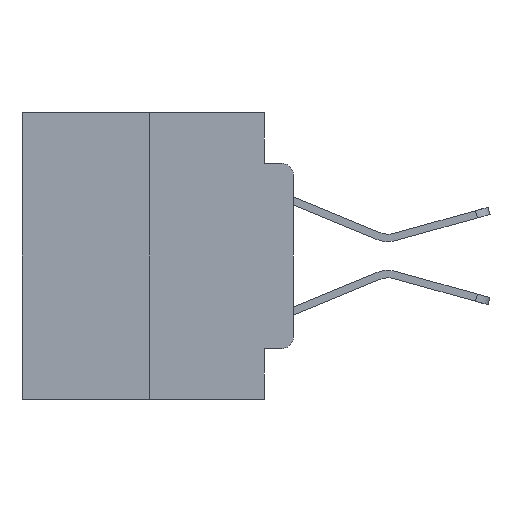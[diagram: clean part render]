
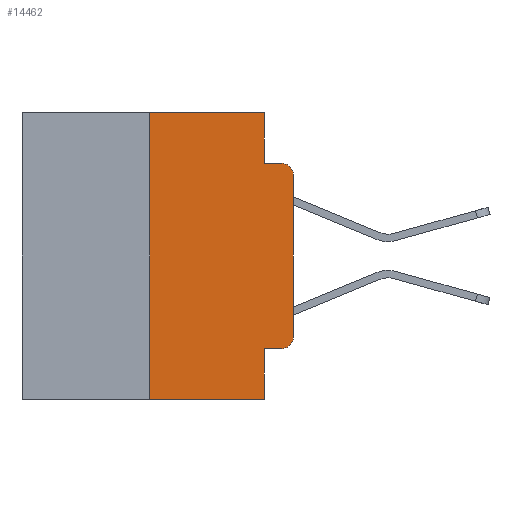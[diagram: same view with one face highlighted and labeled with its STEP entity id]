
A CAD part, left-side view. The second image highlights one B-rep face of the part: STEP entity #14462.
In plain terms, the highlighted planar face has unit normal (-1, 0, 0).
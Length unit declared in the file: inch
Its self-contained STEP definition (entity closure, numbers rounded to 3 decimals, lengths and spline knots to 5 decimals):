
#27 = EDGE_CURVE ( 'NONE', #13425, #13857, #16393, .T. ) ;
#296 = CARTESIAN_POINT ( 'NONE',  ( 0., 0.051, 0. ) ) ;
#343 = VERTEX_POINT ( 'NONE', #26226 ) ;
#1098 = VECTOR ( 'NONE', #14499, 39.37008 ) ;
#1147 = ORIENTED_EDGE ( 'NONE', *, *, #1519, .F. ) ;
#1301 = AXIS2_PLACEMENT_3D ( 'NONE', #14167, #5930, #20452 ) ;
#1519 = EDGE_CURVE ( 'NONE', #9272, #343, #24008, .T. ) ;
#1866 = ORIENTED_EDGE ( 'NONE', *, *, #13255, .T. ) ;
#3032 = AXIS2_PLACEMENT_3D ( 'NONE', #5057, #19577, #7190 ) ;
#3208 = LINE ( 'NONE', #17762, #24667 ) ;
#3587 = ORIENTED_EDGE ( 'NONE', *, *, #12376, .T. ) ;
#4025 = LINE ( 'NONE', #15308, #24775 ) ;
#4399 = CARTESIAN_POINT ( 'NONE',  ( 0., 0.051, -0.0885 ) ) ;
#4735 = CARTESIAN_POINT ( 'NONE',  ( 0., 0.051, 0. ) ) ;
#4945 = DIRECTION ( 'NONE',  ( 0., -1., 0. ) ) ;
#5040 = CARTESIAN_POINT ( 'NONE',  ( 0., 0.051, 0. ) ) ;
#5057 = CARTESIAN_POINT ( 'NONE',  ( 0., 0.02, -0.3915 ) ) ;
#5098 = DIRECTION ( 'NONE',  ( 0., 0., 1. ) ) ;
#5131 = VERTEX_POINT ( 'NONE', #15605 ) ;
#5591 = LINE ( 'NONE', #10428, #15980 ) ;
#5731 = VERTEX_POINT ( 'NONE', #5040 ) ;
#5930 = DIRECTION ( 'NONE',  ( 1., 0., 0. ) ) ;
#7190 = DIRECTION ( 'NONE',  ( 0., 0., -1. ) ) ;
#8165 = DIRECTION ( 'NONE',  ( 0., -1., 0. ) ) ;
#8178 = EDGE_LOOP ( 'NONE', ( #3587, #20245, #9008, #12193, #22541, #1147, #1866, #18371, #22226, #19656 ) ) ;
#8586 = VERTEX_POINT ( 'NONE', #4399 ) ;
#9008 = ORIENTED_EDGE ( 'NONE', *, *, #20384, .F. ) ;
#9272 = VERTEX_POINT ( 'NONE', #16753 ) ;
#9813 = CIRCLE ( 'NONE', #21159, 0.02 ) ;
#10428 = CARTESIAN_POINT ( 'NONE',  ( 0., 0.473, -0.5 ) ) ;
#10515 = VECTOR ( 'NONE', #5098, 39.37008 ) ;
#10891 = VECTOR ( 'NONE', #11155, 39.37008 ) ;
#10939 = LINE ( 'NONE', #18440, #15773 ) ;
#11155 = DIRECTION ( 'NONE',  ( 0., 0., -1. ) ) ;
#11189 = LINE ( 'NONE', #25711, #10515 ) ;
#11396 = CARTESIAN_POINT ( 'NONE',  ( 0., 0., -0.1085 ) ) ;
#11586 = FACE_OUTER_BOUND ( 'NONE', #8178, .T. ) ;
#11681 = VECTOR ( 'NONE', #21353, 39.37008 ) ;
#12111 = CARTESIAN_POINT ( 'NONE',  ( 0., 0.02, -0.1085 ) ) ;
#12193 = ORIENTED_EDGE ( 'NONE', *, *, #18978, .F. ) ;
#12299 = CARTESIAN_POINT ( 'NONE',  ( 0., 0.051, -0.5 ) ) ;
#12376 = EDGE_CURVE ( 'NONE', #23964, #14243, #11189, .T. ) ;
#13035 = CARTESIAN_POINT ( 'NONE',  ( 0., 0.051, -0.4115 ) ) ;
#13255 = EDGE_CURVE ( 'NONE', #9272, #13857, #5591, .T. ) ;
#13425 = VERTEX_POINT ( 'NONE', #13035 ) ;
#13774 = EDGE_CURVE ( 'NONE', #14243, #5131, #9813, .T. ) ;
#13857 = VERTEX_POINT ( 'NONE', #12299 ) ;
#14167 = CARTESIAN_POINT ( 'NONE',  ( 0., 0.473, 0. ) ) ;
#14202 = DIRECTION ( 'NONE',  ( 0., 0., -1. ) ) ;
#14243 = VERTEX_POINT ( 'NONE', #11396 ) ;
#14462 = ADVANCED_FACE ( 'NONE', ( #11586 ), #22387, .F. ) ;
#14478 = EDGE_CURVE ( 'NONE', #343, #5731, #10939, .T. ) ;
#14499 = DIRECTION ( 'NONE',  ( 0., 0., 1. ) ) ;
#14586 = VERTEX_POINT ( 'NONE', #14607 ) ;
#14607 = CARTESIAN_POINT ( 'NONE',  ( 0., 0.02, -0.4115 ) ) ;
#15308 = CARTESIAN_POINT ( 'NONE',  ( 0., 0.051, -0.0885 ) ) ;
#15605 = CARTESIAN_POINT ( 'NONE',  ( 0., 0.02, -0.0885 ) ) ;
#15773 = VECTOR ( 'NONE', #8165, 39.37008 ) ;
#15980 = VECTOR ( 'NONE', #16680, 39.37008 ) ;
#16393 = LINE ( 'NONE', #296, #10891 ) ;
#16680 = DIRECTION ( 'NONE',  ( 0., -1., 0. ) ) ;
#16753 = CARTESIAN_POINT ( 'NONE',  ( 0., 0.25, -0.5 ) ) ;
#17081 = EDGE_CURVE ( 'NONE', #13425, #14586, #3208, .T. ) ;
#17762 = CARTESIAN_POINT ( 'NONE',  ( 0., 0.051, -0.4115 ) ) ;
#18371 = ORIENTED_EDGE ( 'NONE', *, *, #27, .F. ) ;
#18440 = CARTESIAN_POINT ( 'NONE',  ( 0., 0.473, 0. ) ) ;
#18462 = EDGE_CURVE ( 'NONE', #14586, #23964, #19825, .T. ) ;
#18978 = EDGE_CURVE ( 'NONE', #5731, #8586, #22025, .T. ) ;
#19577 = DIRECTION ( 'NONE',  ( -1., 0., 0. ) ) ;
#19656 = ORIENTED_EDGE ( 'NONE', *, *, #18462, .T. ) ;
#19825 = CIRCLE ( 'NONE', #3032, 0.02 ) ;
#20245 = ORIENTED_EDGE ( 'NONE', *, *, #13774, .T. ) ;
#20384 = EDGE_CURVE ( 'NONE', #8586, #5131, #4025, .T. ) ;
#20452 = DIRECTION ( 'NONE',  ( 0., 0., -1. ) ) ;
#21159 = AXIS2_PLACEMENT_3D ( 'NONE', #12111, #26501, #14202 ) ;
#21353 = DIRECTION ( 'NONE',  ( 0., 0., -1. ) ) ;
#21887 = DIRECTION ( 'NONE',  ( 0., -1., 0. ) ) ;
#22025 = LINE ( 'NONE', #4735, #11681 ) ;
#22226 = ORIENTED_EDGE ( 'NONE', *, *, #17081, .T. ) ;
#22387 = PLANE ( 'NONE',  #1301 ) ;
#22541 = ORIENTED_EDGE ( 'NONE', *, *, #14478, .F. ) ;
#23964 = VERTEX_POINT ( 'NONE', #26807 ) ;
#23966 = CARTESIAN_POINT ( 'NONE',  ( 0., 0.25, 0. ) ) ;
#24008 = LINE ( 'NONE', #23966, #1098 ) ;
#24667 = VECTOR ( 'NONE', #21887, 39.37008 ) ;
#24775 = VECTOR ( 'NONE', #4945, 39.37008 ) ;
#25711 = CARTESIAN_POINT ( 'NONE',  ( 0., 0., 0. ) ) ;
#26226 = CARTESIAN_POINT ( 'NONE',  ( 0., 0.25, 0. ) ) ;
#26501 = DIRECTION ( 'NONE',  ( -1., 0., 0. ) ) ;
#26807 = CARTESIAN_POINT ( 'NONE',  ( 0., 0., -0.3915 ) ) ;
